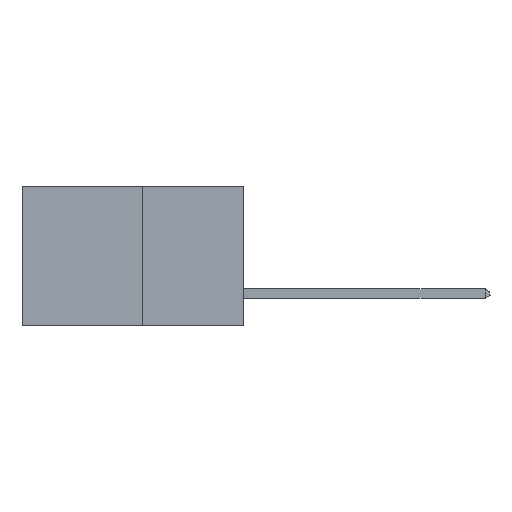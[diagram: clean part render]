
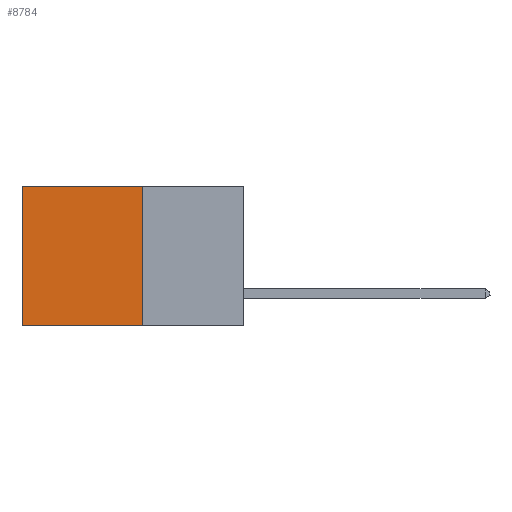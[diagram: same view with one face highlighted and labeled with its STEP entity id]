
A CAD part, left-side view. The second image highlights one B-rep face of the part: STEP entity #8784.
In plain terms, the highlighted planar face has unit normal (-1, 0, 0).
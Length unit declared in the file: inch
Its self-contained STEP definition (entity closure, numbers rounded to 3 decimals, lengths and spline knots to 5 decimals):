
#209 = LINE ( 'NONE', #8493, #2269 ) ;
#759 = DIRECTION ( 'NONE',  ( 0., 0., -1. ) ) ;
#1044 = LINE ( 'NONE', #3811, #7475 ) ;
#1439 = ORIENTED_EDGE ( 'NONE', *, *, #2188, .T. ) ;
#1871 = VERTEX_POINT ( 'NONE', #10390 ) ;
#2188 = EDGE_CURVE ( 'NONE', #1871, #6994, #4299, .T. ) ;
#2269 = VECTOR ( 'NONE', #4492, 39.37008 ) ;
#2407 = CARTESIAN_POINT ( 'NONE',  ( 0.277, 0.59, -0.37 ) ) ;
#2694 = VERTEX_POINT ( 'NONE', #2407 ) ;
#3195 = PLANE ( 'NONE',  #9568 ) ;
#3233 = DIRECTION ( 'NONE',  ( 0., 0., -1. ) ) ;
#3601 = EDGE_LOOP ( 'NONE', ( #5215, #6452, #7051, #1439 ) ) ;
#3718 = VERTEX_POINT ( 'NONE', #8315 ) ;
#3811 = CARTESIAN_POINT ( 'NONE',  ( 0.277, 0.27, -0.37 ) ) ;
#4299 = LINE ( 'NONE', #10304, #6017 ) ;
#4492 = DIRECTION ( 'NONE',  ( 0., 0., -1. ) ) ;
#5215 = ORIENTED_EDGE ( 'NONE', *, *, #9951, .T. ) ;
#5846 = VECTOR ( 'NONE', #759, 39.37008 ) ;
#6017 = VECTOR ( 'NONE', #8508, 39.37008 ) ;
#6091 = LINE ( 'NONE', #10572, #5846 ) ;
#6452 = ORIENTED_EDGE ( 'NONE', *, *, #9460, .F. ) ;
#6994 = VERTEX_POINT ( 'NONE', #10566 ) ;
#7051 = ORIENTED_EDGE ( 'NONE', *, *, #8247, .F. ) ;
#7475 = VECTOR ( 'NONE', #10240, 39.37008 ) ;
#8128 = DIRECTION ( 'NONE',  ( 1., 0., 0. ) ) ;
#8247 = EDGE_CURVE ( 'NONE', #1871, #3718, #6091, .T. ) ;
#8315 = CARTESIAN_POINT ( 'NONE',  ( 0.277, 0.27, -0.37 ) ) ;
#8493 = CARTESIAN_POINT ( 'NONE',  ( 0.277, 0.59, -0.37 ) ) ;
#8508 = DIRECTION ( 'NONE',  ( 0., 1., 0. ) ) ;
#8784 = ADVANCED_FACE ( 'NONE', ( #9923 ), #3195, .F. ) ;
#9460 = EDGE_CURVE ( 'NONE', #3718, #2694, #1044, .T. ) ;
#9568 = AXIS2_PLACEMENT_3D ( 'NONE', #9643, #8128, #3233 ) ;
#9643 = CARTESIAN_POINT ( 'NONE',  ( 0.277, 0.27, -0.37 ) ) ;
#9923 = FACE_OUTER_BOUND ( 'NONE', #3601, .T. ) ;
#9951 = EDGE_CURVE ( 'NONE', #6994, #2694, #209, .T. ) ;
#10240 = DIRECTION ( 'NONE',  ( 0., 1., 0. ) ) ;
#10304 = CARTESIAN_POINT ( 'NONE',  ( 0.277, 0.27, 0. ) ) ;
#10390 = CARTESIAN_POINT ( 'NONE',  ( 0.277, 0.27, 0. ) ) ;
#10566 = CARTESIAN_POINT ( 'NONE',  ( 0.277, 0.59, 0. ) ) ;
#10572 = CARTESIAN_POINT ( 'NONE',  ( 0.277, 0.27, -0.37 ) ) ;
